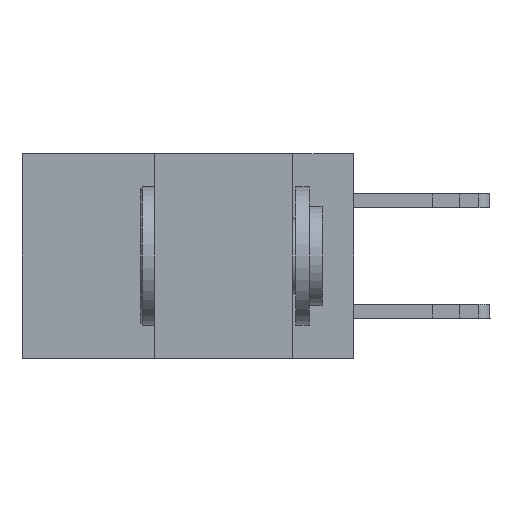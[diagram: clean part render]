
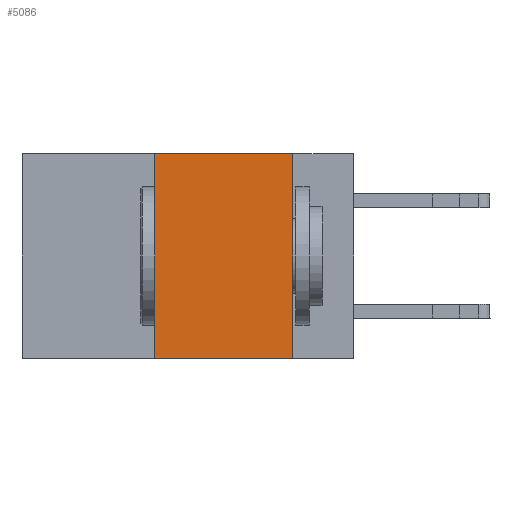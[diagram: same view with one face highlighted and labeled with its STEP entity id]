
A CAD part, left-side view. The second image highlights one B-rep face of the part: STEP entity #5086.
In plain terms, the highlighted planar face has unit normal (-1, 0, 0).
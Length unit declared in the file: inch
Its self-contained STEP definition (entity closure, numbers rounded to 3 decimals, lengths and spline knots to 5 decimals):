
#574 = LINE ( 'NONE', #19675, #14020 ) ;
#1238 = ORIENTED_EDGE ( 'NONE', *, *, #19593, .F. ) ;
#2202 = CARTESIAN_POINT ( 'NONE',  ( 0., 0.6, -0.37 ) ) ;
#2479 = FACE_OUTER_BOUND ( 'NONE', #21103, .T. ) ;
#3621 = VERTEX_POINT ( 'NONE', #8681 ) ;
#4690 = VECTOR ( 'NONE', #16604, 39.37008 ) ;
#5086 = ADVANCED_FACE ( 'NONE', ( #2479 ), #11067, .F. ) ;
#5152 = ORIENTED_EDGE ( 'NONE', *, *, #15314, .F. ) ;
#5495 = VERTEX_POINT ( 'NONE', #7065 ) ;
#5761 = DIRECTION ( 'NONE',  ( 0., 0., -1. ) ) ;
#5925 = VECTOR ( 'NONE', #12138, 39.37008 ) ;
#5973 = DIRECTION ( 'NONE',  ( 0., 0., -1. ) ) ;
#6127 = CARTESIAN_POINT ( 'NONE',  ( 0., 0.6, 0. ) ) ;
#6452 = LINE ( 'NONE', #22470, #5925 ) ;
#7065 = CARTESIAN_POINT ( 'NONE',  ( 0., 0.11, -0.37 ) ) ;
#8514 = LINE ( 'NONE', #2202, #17295 ) ;
#8681 = CARTESIAN_POINT ( 'NONE',  ( 0., 0.36, 0. ) ) ;
#11067 = PLANE ( 'NONE',  #16048 ) ;
#11095 = EDGE_CURVE ( 'NONE', #17253, #5495, #8514, .T. ) ;
#12133 = EDGE_CURVE ( 'NONE', #15444, #5495, #574, .T. ) ;
#12138 = DIRECTION ( 'NONE',  ( 0., 0., 1. ) ) ;
#13479 = LINE ( 'NONE', #6127, #4690 ) ;
#14020 = VECTOR ( 'NONE', #5761, 39.37008 ) ;
#14539 = ORIENTED_EDGE ( 'NONE', *, *, #12133, .F. ) ;
#14721 = CARTESIAN_POINT ( 'NONE',  ( 0., 0.6, 0. ) ) ;
#15232 = CARTESIAN_POINT ( 'NONE',  ( 0., 0.36, -0.37 ) ) ;
#15314 = EDGE_CURVE ( 'NONE', #3621, #15444, #13479, .T. ) ;
#15444 = VERTEX_POINT ( 'NONE', #22135 ) ;
#16048 = AXIS2_PLACEMENT_3D ( 'NONE', #14721, #16435, #5973 ) ;
#16435 = DIRECTION ( 'NONE',  ( 1., 0., 0. ) ) ;
#16604 = DIRECTION ( 'NONE',  ( 0., -1., 0. ) ) ;
#17253 = VERTEX_POINT ( 'NONE', #15232 ) ;
#17295 = VECTOR ( 'NONE', #19627, 39.37008 ) ;
#17341 = ORIENTED_EDGE ( 'NONE', *, *, #11095, .T. ) ;
#19593 = EDGE_CURVE ( 'NONE', #17253, #3621, #6452, .T. ) ;
#19627 = DIRECTION ( 'NONE',  ( 0., -1., 0. ) ) ;
#19675 = CARTESIAN_POINT ( 'NONE',  ( 0., 0.11, 0. ) ) ;
#21103 = EDGE_LOOP ( 'NONE', ( #14539, #5152, #1238, #17341 ) ) ;
#22135 = CARTESIAN_POINT ( 'NONE',  ( 0., 0.11, 0. ) ) ;
#22470 = CARTESIAN_POINT ( 'NONE',  ( 0., 0.36, 0. ) ) ;
